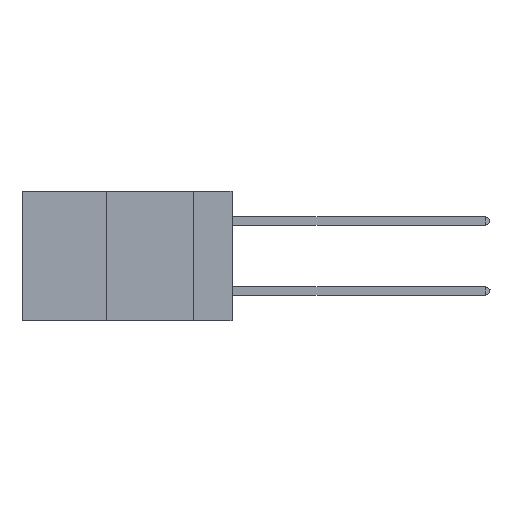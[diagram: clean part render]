
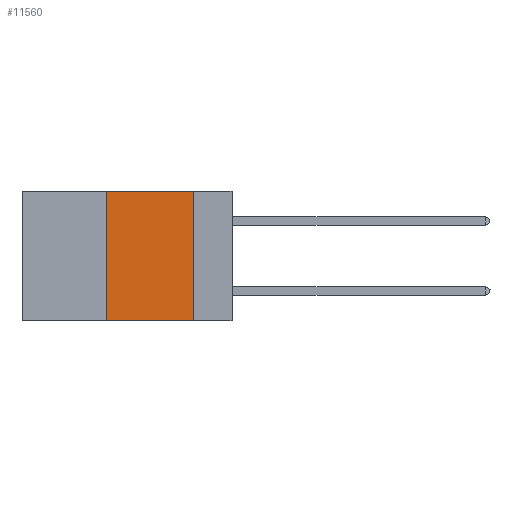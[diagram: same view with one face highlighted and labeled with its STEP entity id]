
A CAD part, left-side view. The second image highlights one B-rep face of the part: STEP entity #11560.
In plain terms, the highlighted planar face has unit normal (-1, 0, 0).
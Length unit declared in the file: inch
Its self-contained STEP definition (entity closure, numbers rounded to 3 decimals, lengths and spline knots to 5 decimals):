
#1505 = ORIENTED_EDGE ( 'NONE', *, *, #3642, .F. ) ;
#2291 = EDGE_CURVE ( 'NONE', #16581, #3540, #16337, .T. ) ;
#2369 = DIRECTION ( 'NONE',  ( 0., -1., 0. ) ) ;
#2418 = DIRECTION ( 'NONE',  ( 0., -1., 0. ) ) ;
#2659 = AXIS2_PLACEMENT_3D ( 'NONE', #12190, #3527, #16169 ) ;
#2974 = CARTESIAN_POINT ( 'NONE',  ( 0., 0.36, -0.37 ) ) ;
#3527 = DIRECTION ( 'NONE',  ( 1., 0., 0. ) ) ;
#3540 = VERTEX_POINT ( 'NONE', #14490 ) ;
#3642 = EDGE_CURVE ( 'NONE', #3540, #4705, #8763, .T. ) ;
#3859 = LINE ( 'NONE', #14095, #7047 ) ;
#4540 = FACE_OUTER_BOUND ( 'NONE', #15023, .T. ) ;
#4705 = VERTEX_POINT ( 'NONE', #13395 ) ;
#4992 = CARTESIAN_POINT ( 'NONE',  ( 0., 0.11, -0.37 ) ) ;
#6122 = DIRECTION ( 'NONE',  ( 0., 0., 1. ) ) ;
#6539 = EDGE_CURVE ( 'NONE', #16581, #14987, #3859, .T. ) ;
#6870 = EDGE_CURVE ( 'NONE', #4705, #14987, #14835, .T. ) ;
#7047 = VECTOR ( 'NONE', #2418, 39.37008 ) ;
#7096 = DIRECTION ( 'NONE',  ( 0., 0., -1. ) ) ;
#7215 = PLANE ( 'NONE',  #2659 ) ;
#8596 = VECTOR ( 'NONE', #6122, 39.37008 ) ;
#8763 = LINE ( 'NONE', #14829, #15912 ) ;
#9897 = ORIENTED_EDGE ( 'NONE', *, *, #6539, .T. ) ;
#10955 = ORIENTED_EDGE ( 'NONE', *, *, #2291, .F. ) ;
#11084 = VECTOR ( 'NONE', #7096, 39.37008 ) ;
#11100 = CARTESIAN_POINT ( 'NONE',  ( 0., 0.11, 0. ) ) ;
#11323 = CARTESIAN_POINT ( 'NONE',  ( 0., 0.36, 0. ) ) ;
#11560 = ADVANCED_FACE ( 'NONE', ( #4540 ), #7215, .F. ) ;
#12190 = CARTESIAN_POINT ( 'NONE',  ( 0., 0.6, 0. ) ) ;
#13395 = CARTESIAN_POINT ( 'NONE',  ( 0., 0.11, 0. ) ) ;
#14095 = CARTESIAN_POINT ( 'NONE',  ( 0., 0.6, -0.37 ) ) ;
#14344 = ORIENTED_EDGE ( 'NONE', *, *, #6870, .F. ) ;
#14490 = CARTESIAN_POINT ( 'NONE',  ( 0., 0.36, 0. ) ) ;
#14829 = CARTESIAN_POINT ( 'NONE',  ( 0., 0.6, 0. ) ) ;
#14835 = LINE ( 'NONE', #11100, #11084 ) ;
#14987 = VERTEX_POINT ( 'NONE', #4992 ) ;
#15023 = EDGE_LOOP ( 'NONE', ( #14344, #1505, #10955, #9897 ) ) ;
#15912 = VECTOR ( 'NONE', #2369, 39.37008 ) ;
#16169 = DIRECTION ( 'NONE',  ( 0., 0., -1. ) ) ;
#16337 = LINE ( 'NONE', #11323, #8596 ) ;
#16581 = VERTEX_POINT ( 'NONE', #2974 ) ;
